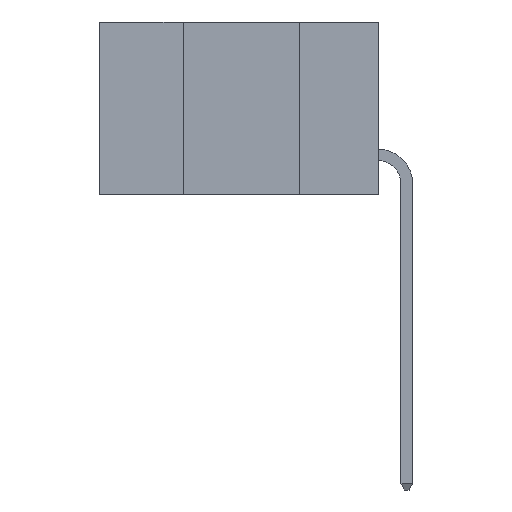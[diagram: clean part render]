
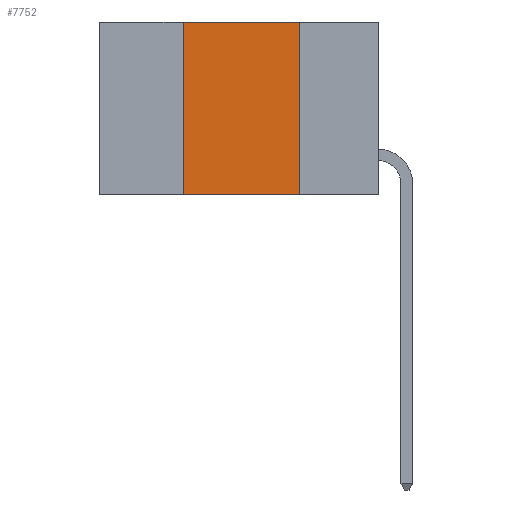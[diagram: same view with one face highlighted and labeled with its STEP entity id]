
A CAD part, left-side view. The second image highlights one B-rep face of the part: STEP entity #7752.
In plain terms, the highlighted planar face has unit normal (-1, 0, 0).
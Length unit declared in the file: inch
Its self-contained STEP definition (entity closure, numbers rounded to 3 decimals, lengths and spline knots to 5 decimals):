
#240 = ORIENTED_EDGE ( 'NONE', *, *, #17314, .F. ) ;
#728 = EDGE_CURVE ( 'NONE', #14829, #6493, #9194, .T. ) ;
#1541 = VERTEX_POINT ( 'NONE', #3056 ) ;
#2402 = LINE ( 'NONE', #9623, #19367 ) ;
#2828 = VECTOR ( 'NONE', #18213, 39.37008 ) ;
#3056 = CARTESIAN_POINT ( 'NONE',  ( 0., 0.17, -0.37 ) ) ;
#4019 = CARTESIAN_POINT ( 'NONE',  ( 0., 0.42, -0.37 ) ) ;
#4868 = VECTOR ( 'NONE', #15138, 39.37008 ) ;
#5036 = VERTEX_POINT ( 'NONE', #14947 ) ;
#5765 = ORIENTED_EDGE ( 'NONE', *, *, #11065, .F. ) ;
#6493 = VERTEX_POINT ( 'NONE', #12732 ) ;
#6526 = EDGE_LOOP ( 'NONE', ( #240, #5765, #20349, #8314 ) ) ;
#7752 = ADVANCED_FACE ( 'NONE', ( #8835 ), #8286, .F. ) ;
#7811 = CARTESIAN_POINT ( 'NONE',  ( 0., 0.42, -0.37 ) ) ;
#8147 = DIRECTION ( 'NONE',  ( 0., 0., -1. ) ) ;
#8167 = DIRECTION ( 'NONE',  ( 1., 0., 0. ) ) ;
#8235 = CARTESIAN_POINT ( 'NONE',  ( 0., 0.6, 0. ) ) ;
#8286 = PLANE ( 'NONE',  #12885 ) ;
#8314 = ORIENTED_EDGE ( 'NONE', *, *, #19439, .T. ) ;
#8835 = FACE_OUTER_BOUND ( 'NONE', #6526, .T. ) ;
#9154 = LINE ( 'NONE', #13438, #17119 ) ;
#9194 = LINE ( 'NONE', #4019, #4868 ) ;
#9623 = CARTESIAN_POINT ( 'NONE',  ( 0., 0.6, 0. ) ) ;
#11065 = EDGE_CURVE ( 'NONE', #6493, #5036, #2402, .T. ) ;
#11983 = LINE ( 'NONE', #18142, #2828 ) ;
#12732 = CARTESIAN_POINT ( 'NONE',  ( 0., 0.42, 0. ) ) ;
#12885 = AXIS2_PLACEMENT_3D ( 'NONE', #8235, #8167, #8147 ) ;
#13438 = CARTESIAN_POINT ( 'NONE',  ( 0., 0.6, -0.37 ) ) ;
#14829 = VERTEX_POINT ( 'NONE', #7811 ) ;
#14947 = CARTESIAN_POINT ( 'NONE',  ( 0., 0.17, 0. ) ) ;
#15046 = DIRECTION ( 'NONE',  ( 0., -1., 0. ) ) ;
#15138 = DIRECTION ( 'NONE',  ( 0., 0., 1. ) ) ;
#17119 = VECTOR ( 'NONE', #15046, 39.37008 ) ;
#17314 = EDGE_CURVE ( 'NONE', #5036, #1541, #11983, .T. ) ;
#18142 = CARTESIAN_POINT ( 'NONE',  ( 0., 0.17, -0.37 ) ) ;
#18213 = DIRECTION ( 'NONE',  ( 0., 0., -1. ) ) ;
#19023 = DIRECTION ( 'NONE',  ( 0., -1., 0. ) ) ;
#19367 = VECTOR ( 'NONE', #19023, 39.37008 ) ;
#19439 = EDGE_CURVE ( 'NONE', #14829, #1541, #9154, .T. ) ;
#20349 = ORIENTED_EDGE ( 'NONE', *, *, #728, .F. ) ;
